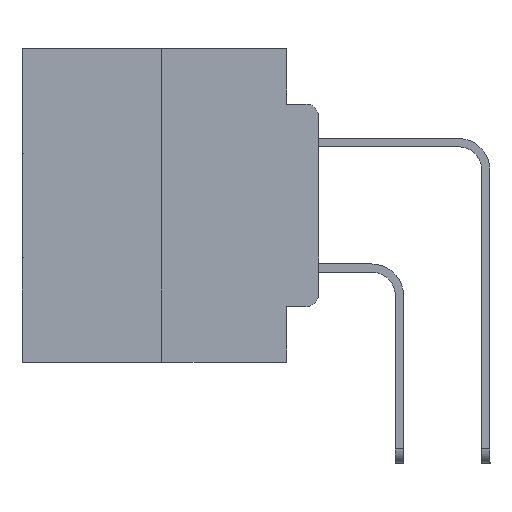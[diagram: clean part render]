
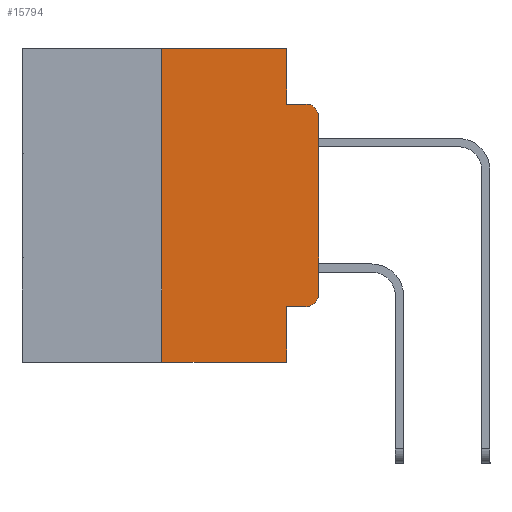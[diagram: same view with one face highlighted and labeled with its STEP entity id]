
A CAD part, left-side view. The second image highlights one B-rep face of the part: STEP entity #15794.
In plain terms, the highlighted planar face has unit normal (-1, 0, 0).
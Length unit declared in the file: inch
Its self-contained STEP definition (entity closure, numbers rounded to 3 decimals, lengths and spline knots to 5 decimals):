
#59 = EDGE_CURVE ( 'NONE', #29742, #2767, #17628, .T. ) ;
#216 = DIRECTION ( 'NONE',  ( -1., 0., 0. ) ) ;
#433 = VERTEX_POINT ( 'NONE', #21234 ) ;
#1435 = EDGE_CURVE ( 'NONE', #4386, #10488, #24554, .T. ) ;
#1479 = ORIENTED_EDGE ( 'NONE', *, *, #17833, .T. ) ;
#1919 = DIRECTION ( 'NONE',  ( 0., 0., 1. ) ) ;
#1950 = PLANE ( 'NONE',  #3264 ) ;
#2022 = VECTOR ( 'NONE', #26598, 39.37008 ) ;
#2096 = EDGE_CURVE ( 'NONE', #10488, #433, #21726, .T. ) ;
#2566 = ORIENTED_EDGE ( 'NONE', *, *, #19259, .T. ) ;
#2614 = CARTESIAN_POINT ( 'NONE',  ( 0., 0.25, 0. ) ) ;
#2767 = VERTEX_POINT ( 'NONE', #15646 ) ;
#3264 = AXIS2_PLACEMENT_3D ( 'NONE', #6770, #18918, #4446 ) ;
#4084 = VERTEX_POINT ( 'NONE', #27058 ) ;
#4267 = LINE ( 'NONE', #24833, #9989 ) ;
#4386 = VERTEX_POINT ( 'NONE', #6646 ) ;
#4446 = DIRECTION ( 'NONE',  ( 0., 0., -1. ) ) ;
#4532 = ORIENTED_EDGE ( 'NONE', *, *, #8665, .F. ) ;
#4641 = FACE_OUTER_BOUND ( 'NONE', #12993, .T. ) ;
#4778 = CARTESIAN_POINT ( 'NONE',  ( 0., 0.051, 0. ) ) ;
#4888 = ORIENTED_EDGE ( 'NONE', *, *, #24061, .T. ) ;
#4936 = VERTEX_POINT ( 'NONE', #25362 ) ;
#5078 = DIRECTION ( 'NONE',  ( 0., 0., 1. ) ) ;
#5154 = LINE ( 'NONE', #9210, #11668 ) ;
#5671 = DIRECTION ( 'NONE',  ( 0., -1., 0. ) ) ;
#6646 = CARTESIAN_POINT ( 'NONE',  ( 0., 0.051, -0.4115 ) ) ;
#6770 = CARTESIAN_POINT ( 'NONE',  ( 0., 0.473, 0. ) ) ;
#6798 = ORIENTED_EDGE ( 'NONE', *, *, #25910, .F. ) ;
#7303 = EDGE_CURVE ( 'NONE', #4084, #29742, #19939, .T. ) ;
#7453 = DIRECTION ( 'NONE',  ( 0., -1., 0. ) ) ;
#7830 = AXIS2_PLACEMENT_3D ( 'NONE', #14882, #216, #17292 ) ;
#8248 = CIRCLE ( 'NONE', #7830, 0.02 ) ;
#8665 = EDGE_CURVE ( 'NONE', #22651, #4936, #14255, .T. ) ;
#9210 = CARTESIAN_POINT ( 'NONE',  ( 0., 0., 0. ) ) ;
#9403 = CARTESIAN_POINT ( 'NONE',  ( 0., 0.051, -0.0885 ) ) ;
#9930 = CARTESIAN_POINT ( 'NONE',  ( 0., 0.02, -0.4115 ) ) ;
#9989 = VECTOR ( 'NONE', #13012, 39.37008 ) ;
#10036 = CARTESIAN_POINT ( 'NONE',  ( 0., 0.051, -0.0885 ) ) ;
#10058 = CARTESIAN_POINT ( 'NONE',  ( 0., 0., -0.1085 ) ) ;
#10488 = VERTEX_POINT ( 'NONE', #9930 ) ;
#10660 = EDGE_CURVE ( 'NONE', #4386, #24072, #4267, .T. ) ;
#11668 = VECTOR ( 'NONE', #1919, 39.37008 ) ;
#11986 = VECTOR ( 'NONE', #28628, 39.37008 ) ;
#12927 = ORIENTED_EDGE ( 'NONE', *, *, #59, .F. ) ;
#12993 = EDGE_LOOP ( 'NONE', ( #2566, #4888, #4532, #6798, #12927, #17838, #1479, #14859, #28235, #24176 ) ) ;
#13012 = DIRECTION ( 'NONE',  ( 0., 0., -1. ) ) ;
#14033 = LINE ( 'NONE', #20109, #21085 ) ;
#14217 = CARTESIAN_POINT ( 'NONE',  ( 0., 0.473, 0. ) ) ;
#14255 = LINE ( 'NONE', #10036, #2022 ) ;
#14859 = ORIENTED_EDGE ( 'NONE', *, *, #10660, .F. ) ;
#14882 = CARTESIAN_POINT ( 'NONE',  ( 0., 0.02, -0.1085 ) ) ;
#15646 = CARTESIAN_POINT ( 'NONE',  ( 0., 0.051, 0. ) ) ;
#15794 = ADVANCED_FACE ( 'NONE', ( #4641 ), #1950, .F. ) ;
#16895 = VECTOR ( 'NONE', #7453, 39.37008 ) ;
#16973 = VECTOR ( 'NONE', #5078, 39.37008 ) ;
#17292 = DIRECTION ( 'NONE',  ( 0., 0., -1. ) ) ;
#17580 = CARTESIAN_POINT ( 'NONE',  ( 0., 0.051, -0.4115 ) ) ;
#17628 = LINE ( 'NONE', #14217, #16895 ) ;
#17690 = DIRECTION ( 'NONE',  ( 0., -1., 0. ) ) ;
#17833 = EDGE_CURVE ( 'NONE', #4084, #24072, #14033, .T. ) ;
#17838 = ORIENTED_EDGE ( 'NONE', *, *, #7303, .F. ) ;
#18279 = VECTOR ( 'NONE', #17690, 39.37008 ) ;
#18352 = LINE ( 'NONE', #4778, #11986 ) ;
#18918 = DIRECTION ( 'NONE',  ( 1., 0., 0. ) ) ;
#19259 = EDGE_CURVE ( 'NONE', #433, #19477, #5154, .T. ) ;
#19477 = VERTEX_POINT ( 'NONE', #10058 ) ;
#19939 = LINE ( 'NONE', #2614, #16973 ) ;
#20109 = CARTESIAN_POINT ( 'NONE',  ( 0., 0.473, -0.5 ) ) ;
#21085 = VECTOR ( 'NONE', #5671, 39.37008 ) ;
#21234 = CARTESIAN_POINT ( 'NONE',  ( 0., 0., -0.3915 ) ) ;
#21726 = CIRCLE ( 'NONE', #27125, 0.02 ) ;
#22651 = VERTEX_POINT ( 'NONE', #9403 ) ;
#23361 = CARTESIAN_POINT ( 'NONE',  ( 0., 0.25, 0. ) ) ;
#24061 = EDGE_CURVE ( 'NONE', #19477, #4936, #8248, .T. ) ;
#24072 = VERTEX_POINT ( 'NONE', #24404 ) ;
#24176 = ORIENTED_EDGE ( 'NONE', *, *, #2096, .T. ) ;
#24404 = CARTESIAN_POINT ( 'NONE',  ( 0., 0.051, -0.5 ) ) ;
#24554 = LINE ( 'NONE', #17580, #18279 ) ;
#24692 = DIRECTION ( 'NONE',  ( 0., 0., -1. ) ) ;
#24833 = CARTESIAN_POINT ( 'NONE',  ( 0., 0.051, 0. ) ) ;
#25362 = CARTESIAN_POINT ( 'NONE',  ( 0., 0.02, -0.0885 ) ) ;
#25910 = EDGE_CURVE ( 'NONE', #2767, #22651, #18352, .T. ) ;
#26155 = CARTESIAN_POINT ( 'NONE',  ( 0., 0.02, -0.3915 ) ) ;
#26598 = DIRECTION ( 'NONE',  ( 0., -1., 0. ) ) ;
#26764 = DIRECTION ( 'NONE',  ( -1., 0., 0. ) ) ;
#27058 = CARTESIAN_POINT ( 'NONE',  ( 0., 0.25, -0.5 ) ) ;
#27125 = AXIS2_PLACEMENT_3D ( 'NONE', #26155, #26764, #24692 ) ;
#28235 = ORIENTED_EDGE ( 'NONE', *, *, #1435, .T. ) ;
#28628 = DIRECTION ( 'NONE',  ( 0., 0., -1. ) ) ;
#29742 = VERTEX_POINT ( 'NONE', #23361 ) ;
